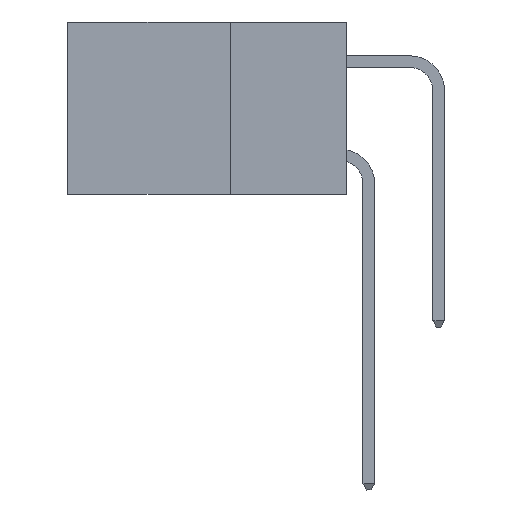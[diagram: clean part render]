
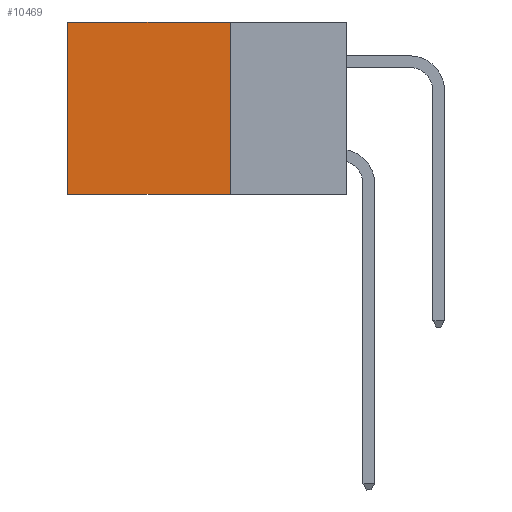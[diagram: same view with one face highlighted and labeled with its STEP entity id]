
A CAD part, left-side view. The second image highlights one B-rep face of the part: STEP entity #10469.
In plain terms, the highlighted planar face has unit normal (-1, 0, 0).
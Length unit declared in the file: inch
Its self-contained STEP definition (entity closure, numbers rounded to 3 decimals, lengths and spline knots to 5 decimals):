
#482 = VERTEX_POINT ( 'NONE', #12671 ) ;
#688 = DIRECTION ( 'NONE',  ( 1., 0., 0. ) ) ;
#798 = CARTESIAN_POINT ( 'NONE',  ( 0.2875, 0.6, -0.37 ) ) ;
#917 = ORIENTED_EDGE ( 'NONE', *, *, #1931, .T. ) ;
#1931 = EDGE_CURVE ( 'NONE', #10726, #482, #9969, .T. ) ;
#2355 = VECTOR ( 'NONE', #2707, 39.37008 ) ;
#2671 = VECTOR ( 'NONE', #10090, 39.37008 ) ;
#2676 = ORIENTED_EDGE ( 'NONE', *, *, #5498, .T. ) ;
#2707 = DIRECTION ( 'NONE',  ( 0., 0., -1. ) ) ;
#4092 = DIRECTION ( 'NONE',  ( 0., 1., 0. ) ) ;
#4190 = CARTESIAN_POINT ( 'NONE',  ( 0.2875, 0.25, 0. ) ) ;
#4535 = ORIENTED_EDGE ( 'NONE', *, *, #5079, .F. ) ;
#4983 = CARTESIAN_POINT ( 'NONE',  ( 0.2875, 0.25, -0.37 ) ) ;
#5079 = EDGE_CURVE ( 'NONE', #9723, #5783, #14010, .T. ) ;
#5100 = CARTESIAN_POINT ( 'NONE',  ( 0.2875, 0.25, 0. ) ) ;
#5391 = FACE_OUTER_BOUND ( 'NONE', #8394, .T. ) ;
#5498 = EDGE_CURVE ( 'NONE', #482, #5783, #5547, .T. ) ;
#5547 = LINE ( 'NONE', #5696, #2671 ) ;
#5561 = VECTOR ( 'NONE', #6082, 39.37008 ) ;
#5696 = CARTESIAN_POINT ( 'NONE',  ( 0.2875, 0.6, 0. ) ) ;
#5783 = VERTEX_POINT ( 'NONE', #798 ) ;
#6082 = DIRECTION ( 'NONE',  ( 0., 1., 0. ) ) ;
#6205 = AXIS2_PLACEMENT_3D ( 'NONE', #5100, #688, #8430 ) ;
#6341 = VECTOR ( 'NONE', #4092, 39.37008 ) ;
#6795 = CARTESIAN_POINT ( 'NONE',  ( 0.2875, 0.25, 0. ) ) ;
#7329 = PLANE ( 'NONE',  #6205 ) ;
#8394 = EDGE_LOOP ( 'NONE', ( #2676, #4535, #12994, #917 ) ) ;
#8430 = DIRECTION ( 'NONE',  ( 0., 0., -1. ) ) ;
#9247 = CARTESIAN_POINT ( 'NONE',  ( 0.2875, 0.25, 0. ) ) ;
#9406 = CARTESIAN_POINT ( 'NONE',  ( 0.2875, 0.25, -0.37 ) ) ;
#9723 = VERTEX_POINT ( 'NONE', #9406 ) ;
#9969 = LINE ( 'NONE', #4190, #6341 ) ;
#10090 = DIRECTION ( 'NONE',  ( 0., 0., -1. ) ) ;
#10313 = EDGE_CURVE ( 'NONE', #10726, #9723, #13696, .T. ) ;
#10469 = ADVANCED_FACE ( 'NONE', ( #5391 ), #7329, .F. ) ;
#10726 = VERTEX_POINT ( 'NONE', #6795 ) ;
#12671 = CARTESIAN_POINT ( 'NONE',  ( 0.2875, 0.6, 0. ) ) ;
#12994 = ORIENTED_EDGE ( 'NONE', *, *, #10313, .F. ) ;
#13696 = LINE ( 'NONE', #9247, #2355 ) ;
#14010 = LINE ( 'NONE', #4983, #5561 ) ;
